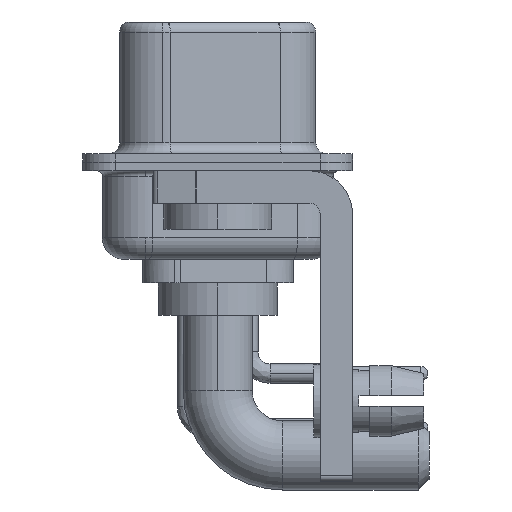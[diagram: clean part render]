
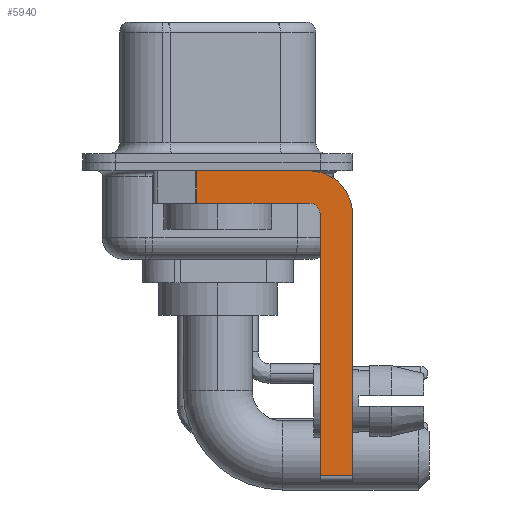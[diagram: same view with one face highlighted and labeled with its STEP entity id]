
A CAD part, left-side view. The second image highlights one B-rep face of the part: STEP entity #5940.
In plain terms, the highlighted planar face has unit normal (-1, 0, 0).
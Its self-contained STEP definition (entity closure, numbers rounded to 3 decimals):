
#975 = ORIENTED_EDGE ( 'NONE', *, *, #25188, .F. ) ;
#1636 = EDGE_CURVE ( 'NONE', #13407, #27706, #20961, .T. ) ;
#1983 = FACE_OUTER_BOUND ( 'NONE', #7371, .T. ) ;
#2013 = EDGE_CURVE ( 'NONE', #20752, #24162, #23824, .T. ) ;
#2132 = DIRECTION ( 'NONE',  ( 0., 0., -1. ) ) ;
#2934 = EDGE_CURVE ( 'NONE', #13407, #3958, #7447, .T. ) ;
#2949 = DIRECTION ( 'NONE',  ( 1., 0., 0. ) ) ;
#3021 = DIRECTION ( 'NONE',  ( 0., 0., 1. ) ) ;
#3221 = CARTESIAN_POINT ( 'NONE',  ( -2.9, -6.25, -2.4 ) ) ;
#3477 = ORIENTED_EDGE ( 'NONE', *, *, #20831, .F. ) ;
#3958 = VERTEX_POINT ( 'NONE', #19828 ) ;
#4142 = EDGE_CURVE ( 'NONE', #17506, #27057, #6727, .T. ) ;
#4310 = DIRECTION ( 'NONE',  ( 0., -1., 0. ) ) ;
#4511 = CIRCLE ( 'NONE', #21756, 2. ) ;
#5192 = LINE ( 'NONE', #14604, #22315 ) ;
#5940 = ADVANCED_FACE ( 'NONE', ( #1983 ), #11381, .F. ) ;
#6727 = CIRCLE ( 'NONE', #28404, 0.5 ) ;
#7371 = EDGE_LOOP ( 'NONE', ( #11156, #15504, #3477, #8867, #23981, #11266, #975, #14742 ) ) ;
#7447 = LINE ( 'NONE', #9449, #23343 ) ;
#8404 = EDGE_CURVE ( 'NONE', #20752, #17506, #5192, .T. ) ;
#8570 = CARTESIAN_POINT ( 'NONE',  ( -2.9, -4.75, -2.4 ) ) ;
#8867 = ORIENTED_EDGE ( 'NONE', *, *, #4142, .F. ) ;
#9185 = CARTESIAN_POINT ( 'NONE',  ( -2.9, -4.25, -2.4 ) ) ;
#9449 = CARTESIAN_POINT ( 'NONE',  ( -2.9, 0.978, -1.9 ) ) ;
#9872 = DIRECTION ( 'NONE',  ( 0., 0., -1. ) ) ;
#11156 = ORIENTED_EDGE ( 'NONE', *, *, #1636, .F. ) ;
#11266 = ORIENTED_EDGE ( 'NONE', *, *, #2013, .T. ) ;
#11337 = DIRECTION ( 'NONE',  ( 0., 0., 1. ) ) ;
#11381 = PLANE ( 'NONE',  #22280 ) ;
#12058 = EDGE_CURVE ( 'NONE', #27706, #14281, #4511, .T. ) ;
#12374 = DIRECTION ( 'NONE',  ( -1., 0., 0. ) ) ;
#13270 = VECTOR ( 'NONE', #14131, 1000. ) ;
#13407 = VERTEX_POINT ( 'NONE', #24101 ) ;
#13860 = DIRECTION ( 'NONE',  ( 1., 0., 0. ) ) ;
#14131 = DIRECTION ( 'NONE',  ( 0., 1., 0. ) ) ;
#14281 = VERTEX_POINT ( 'NONE', #24373 ) ;
#14604 = CARTESIAN_POINT ( 'NONE',  ( -2.9, -4.75, -14.8 ) ) ;
#14742 = ORIENTED_EDGE ( 'NONE', *, *, #12058, .F. ) ;
#15504 = ORIENTED_EDGE ( 'NONE', *, *, #2934, .T. ) ;
#16539 = DIRECTION ( 'NONE',  ( 0., 0., -1. ) ) ;
#17480 = CARTESIAN_POINT ( 'NONE',  ( -2.9, -6.25, -14.55 ) ) ;
#17499 = VECTOR ( 'NONE', #9872, 1000. ) ;
#17506 = VERTEX_POINT ( 'NONE', #8570 ) ;
#17577 = DIRECTION ( 'NONE',  ( 0., 0., -1. ) ) ;
#18293 = CARTESIAN_POINT ( 'NONE',  ( -2.9, -4.25, -1.9 ) ) ;
#18479 = CARTESIAN_POINT ( 'NONE',  ( -2.9, -4.25, -0.4 ) ) ;
#18487 = CARTESIAN_POINT ( 'NONE',  ( -2.9, -4.25, -2.4 ) ) ;
#19299 = CARTESIAN_POINT ( 'NONE',  ( -2.9, -4.25, -2.4 ) ) ;
#19418 = LINE ( 'NONE', #3221, #17499 ) ;
#19828 = CARTESIAN_POINT ( 'NONE',  ( -2.9, 0.978, -1.9 ) ) ;
#20752 = VERTEX_POINT ( 'NONE', #22172 ) ;
#20831 = EDGE_CURVE ( 'NONE', #27057, #3958, #28020, .T. ) ;
#20961 = LINE ( 'NONE', #25439, #27994 ) ;
#21513 = DIRECTION ( 'NONE',  ( 0., -1., 0. ) ) ;
#21756 = AXIS2_PLACEMENT_3D ( 'NONE', #19299, #2949, #17577 ) ;
#22172 = CARTESIAN_POINT ( 'NONE',  ( -2.9, -4.75, -14.55 ) ) ;
#22280 = AXIS2_PLACEMENT_3D ( 'NONE', #18487, #13860, #2132 ) ;
#22315 = VECTOR ( 'NONE', #3021, 1000. ) ;
#23343 = VECTOR ( 'NONE', #16539, 1000. ) ;
#23824 = LINE ( 'NONE', #28459, #25568 ) ;
#23981 = ORIENTED_EDGE ( 'NONE', *, *, #8404, .F. ) ;
#24101 = CARTESIAN_POINT ( 'NONE',  ( -2.9, 0.978, -0.4 ) ) ;
#24162 = VERTEX_POINT ( 'NONE', #17480 ) ;
#24373 = CARTESIAN_POINT ( 'NONE',  ( -2.9, -6.25, -2.4 ) ) ;
#25188 = EDGE_CURVE ( 'NONE', #14281, #24162, #19418, .T. ) ;
#25439 = CARTESIAN_POINT ( 'NONE',  ( -2.9, 3., -0.4 ) ) ;
#25568 = VECTOR ( 'NONE', #21513, 1000. ) ;
#27057 = VERTEX_POINT ( 'NONE', #29322 ) ;
#27706 = VERTEX_POINT ( 'NONE', #18479 ) ;
#27994 = VECTOR ( 'NONE', #4310, 1000. ) ;
#28020 = LINE ( 'NONE', #18293, #13270 ) ;
#28404 = AXIS2_PLACEMENT_3D ( 'NONE', #9185, #12374, #11337 ) ;
#28459 = CARTESIAN_POINT ( 'NONE',  ( -2.9, -4.25, -14.55 ) ) ;
#29322 = CARTESIAN_POINT ( 'NONE',  ( -2.9, -4.25, -1.9 ) ) ;
